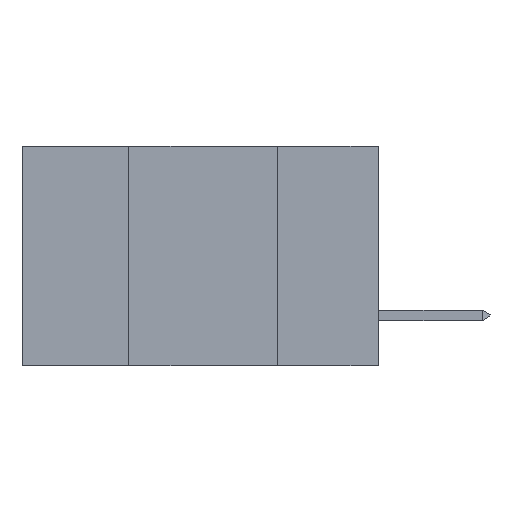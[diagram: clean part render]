
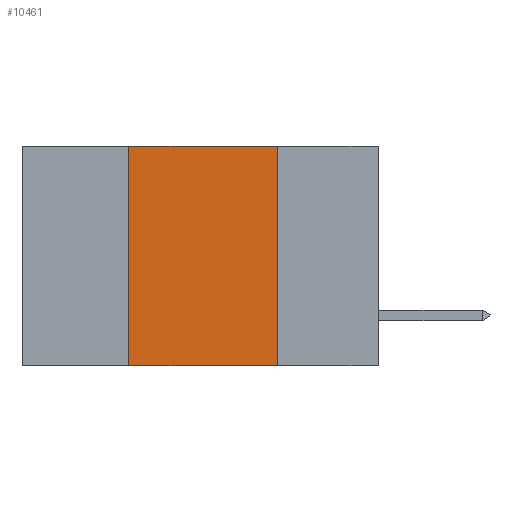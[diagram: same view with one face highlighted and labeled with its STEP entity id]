
A CAD part, left-side view. The second image highlights one B-rep face of the part: STEP entity #10461.
In plain terms, the highlighted planar face has unit normal (-1, 0, 0).
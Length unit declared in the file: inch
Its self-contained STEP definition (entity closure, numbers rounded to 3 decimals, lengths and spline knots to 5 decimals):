
#80 = CARTESIAN_POINT ( 'NONE',  ( 0., 0.17, 0. ) ) ;
#454 = ORIENTED_EDGE ( 'NONE', *, *, #727, .F. ) ;
#727 = EDGE_CURVE ( 'NONE', #10621, #8414, #7511, .T. ) ;
#800 = FACE_OUTER_BOUND ( 'NONE', #3693, .T. ) ;
#1364 = ORIENTED_EDGE ( 'NONE', *, *, #7417, .T. ) ;
#1831 = AXIS2_PLACEMENT_3D ( 'NONE', #2855, #12327, #13525 ) ;
#1944 = DIRECTION ( 'NONE',  ( 0., 0., 1. ) ) ;
#2209 = LINE ( 'NONE', #3498, #11454 ) ;
#2855 = CARTESIAN_POINT ( 'NONE',  ( 0., 0.6, 0. ) ) ;
#2935 = VECTOR ( 'NONE', #12455, 39.37008 ) ;
#2956 = VERTEX_POINT ( 'NONE', #12498 ) ;
#2986 = CARTESIAN_POINT ( 'NONE',  ( 0., 0.42, -0.37 ) ) ;
#3498 = CARTESIAN_POINT ( 'NONE',  ( 0., 0.17, -0.37 ) ) ;
#3693 = EDGE_LOOP ( 'NONE', ( #7310, #11654, #454, #1364 ) ) ;
#3898 = PLANE ( 'NONE',  #1831 ) ;
#3983 = LINE ( 'NONE', #11642, #7835 ) ;
#4849 = EDGE_CURVE ( 'NONE', #5900, #2956, #2209, .T. ) ;
#5900 = VERTEX_POINT ( 'NONE', #80 ) ;
#6119 = LINE ( 'NONE', #9079, #2935 ) ;
#6672 = VECTOR ( 'NONE', #1944, 39.37008 ) ;
#7310 = ORIENTED_EDGE ( 'NONE', *, *, #4849, .F. ) ;
#7417 = EDGE_CURVE ( 'NONE', #10621, #2956, #3983, .T. ) ;
#7511 = LINE ( 'NONE', #2986, #6672 ) ;
#7835 = VECTOR ( 'NONE', #11597, 39.37008 ) ;
#8414 = VERTEX_POINT ( 'NONE', #10389 ) ;
#9079 = CARTESIAN_POINT ( 'NONE',  ( 0., 0.6, 0. ) ) ;
#9949 = DIRECTION ( 'NONE',  ( 0., 0., -1. ) ) ;
#10389 = CARTESIAN_POINT ( 'NONE',  ( 0., 0.42, 0. ) ) ;
#10461 = ADVANCED_FACE ( 'NONE', ( #800 ), #3898, .F. ) ;
#10621 = VERTEX_POINT ( 'NONE', #13061 ) ;
#11454 = VECTOR ( 'NONE', #9949, 39.37008 ) ;
#11597 = DIRECTION ( 'NONE',  ( 0., -1., 0. ) ) ;
#11642 = CARTESIAN_POINT ( 'NONE',  ( 0., 0.6, -0.37 ) ) ;
#11654 = ORIENTED_EDGE ( 'NONE', *, *, #11767, .F. ) ;
#11767 = EDGE_CURVE ( 'NONE', #8414, #5900, #6119, .T. ) ;
#12327 = DIRECTION ( 'NONE',  ( 1., 0., 0. ) ) ;
#12455 = DIRECTION ( 'NONE',  ( 0., -1., 0. ) ) ;
#12498 = CARTESIAN_POINT ( 'NONE',  ( 0., 0.17, -0.37 ) ) ;
#13061 = CARTESIAN_POINT ( 'NONE',  ( 0., 0.42, -0.37 ) ) ;
#13525 = DIRECTION ( 'NONE',  ( 0., 0., -1. ) ) ;
